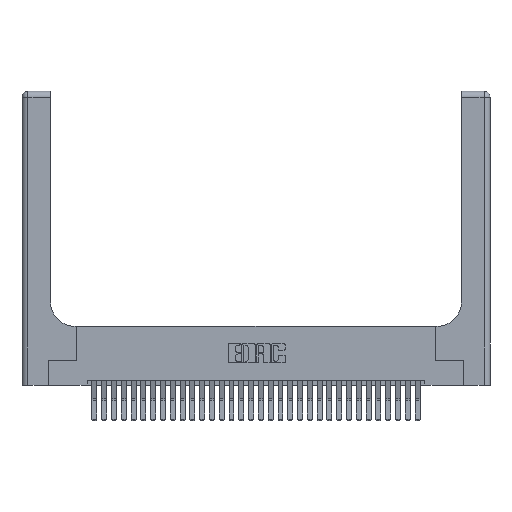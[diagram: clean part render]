
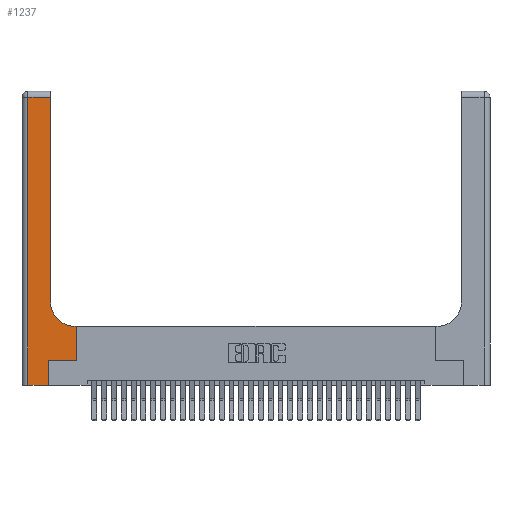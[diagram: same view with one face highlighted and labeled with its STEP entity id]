
A CAD part, top view. The second image highlights one B-rep face of the part: STEP entity #1237.
In plain terms, the highlighted planar face has unit normal (0, 0, 1).
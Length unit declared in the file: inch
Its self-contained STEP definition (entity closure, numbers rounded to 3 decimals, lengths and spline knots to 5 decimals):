
#250 = DIRECTION ( 'NONE',  ( 0., 1., 0. ) ) ;
#1136 = ORIENTED_EDGE ( 'NONE', *, *, #24764, .T. ) ;
#1237 = ADVANCED_FACE ( 'NONE', ( #21443 ), #8126, .F. ) ;
#2355 = CARTESIAN_POINT ( 'NONE',  ( 0.06, 0., 0.37 ) ) ;
#3343 = CARTESIAN_POINT ( 'NONE',  ( 0.06, 3., 0.37 ) ) ;
#3361 = EDGE_CURVE ( 'NONE', #28414, #32316, #3739, .T. ) ;
#3411 = LINE ( 'NONE', #3343, #25801 ) ;
#3739 = LINE ( 'NONE', #21018, #9741 ) ;
#3872 = EDGE_CURVE ( 'NONE', #28305, #20865, #8903, .T. ) ;
#4763 = VERTEX_POINT ( 'NONE', #10488 ) ;
#5432 = VERTEX_POINT ( 'NONE', #10334 ) ;
#5720 = DIRECTION ( 'NONE',  ( -1., 0., 0. ) ) ;
#6015 = EDGE_CURVE ( 'NONE', #20865, #5432, #26299, .T. ) ;
#6050 = LINE ( 'NONE', #10489, #30754 ) ;
#7619 = CARTESIAN_POINT ( 'NONE',  ( 0.269, 0., 0.37 ) ) ;
#7995 = DIRECTION ( 'NONE',  ( -1., 0., 0. ) ) ;
#8056 = DIRECTION ( 'NONE',  ( 0., 0., -1. ) ) ;
#8109 = CIRCLE ( 'NONE', #25505, 0.25 ) ;
#8126 = PLANE ( 'NONE',  #14639 ) ;
#8235 = CARTESIAN_POINT ( 'NONE',  ( 0.5585, 0.25, 0.37 ) ) ;
#8295 = CARTESIAN_POINT ( 'NONE',  ( 0., 3., 0.37 ) ) ;
#8903 = LINE ( 'NONE', #18046, #21658 ) ;
#9468 = ORIENTED_EDGE ( 'NONE', *, *, #23915, .T. ) ;
#9731 = CARTESIAN_POINT ( 'NONE',  ( 0.5585, 0.25, 0.37 ) ) ;
#9741 = VECTOR ( 'NONE', #23598, 39.37008 ) ;
#9792 = ORIENTED_EDGE ( 'NONE', *, *, #22932, .T. ) ;
#10334 = CARTESIAN_POINT ( 'NONE',  ( 0.5585, 0.6, 0.37 ) ) ;
#10488 = CARTESIAN_POINT ( 'NONE',  ( 0.06, 2.94, 0.37 ) ) ;
#10489 = CARTESIAN_POINT ( 'NONE',  ( 0.2915, 3., 0.37 ) ) ;
#12262 = CARTESIAN_POINT ( 'NONE',  ( 0.269, 0.25, 0.37 ) ) ;
#12345 = DIRECTION ( 'NONE',  ( 0., 1., 0. ) ) ;
#12402 = EDGE_LOOP ( 'NONE', ( #27094, #12932, #9468, #13597, #1136, #17725, #28797, #9792, #27145 ) ) ;
#12486 = CARTESIAN_POINT ( 'NONE',  ( 0.2915, 0.85, 0.37 ) ) ;
#12932 = ORIENTED_EDGE ( 'NONE', *, *, #32480, .T. ) ;
#13597 = ORIENTED_EDGE ( 'NONE', *, *, #3361, .T. ) ;
#14222 = CARTESIAN_POINT ( 'NONE',  ( 0.2915, 2.94, 0.37 ) ) ;
#14639 = AXIS2_PLACEMENT_3D ( 'NONE', #8295, #8056, #7995 ) ;
#15144 = DIRECTION ( 'NONE',  ( 0., 0., -1. ) ) ;
#15532 = DIRECTION ( 'NONE',  ( 1., 0., 0. ) ) ;
#16911 = CARTESIAN_POINT ( 'NONE',  ( 0.5415, 0.6, 0.37 ) ) ;
#17421 = VECTOR ( 'NONE', #32781, 39.37008 ) ;
#17451 = CARTESIAN_POINT ( 'NONE',  ( 0.269, 0., 0.37 ) ) ;
#17725 = ORIENTED_EDGE ( 'NONE', *, *, #3872, .T. ) ;
#18046 = CARTESIAN_POINT ( 'NONE',  ( 0.269, 0.25, 0.37 ) ) ;
#18403 = CARTESIAN_POINT ( 'NONE',  ( 0., 2.94, 0.37 ) ) ;
#20865 = VERTEX_POINT ( 'NONE', #8235 ) ;
#21018 = CARTESIAN_POINT ( 'NONE',  ( 0., 0., 0.37 ) ) ;
#21443 = FACE_OUTER_BOUND ( 'NONE', #12402, .T. ) ;
#21658 = VECTOR ( 'NONE', #15532, 39.37008 ) ;
#21734 = VERTEX_POINT ( 'NONE', #14222 ) ;
#22932 = EDGE_CURVE ( 'NONE', #5432, #24723, #30987, .T. ) ;
#23598 = DIRECTION ( 'NONE',  ( 1., 0., 0. ) ) ;
#23786 = DIRECTION ( 'NONE',  ( 0., -1., 0. ) ) ;
#23915 = EDGE_CURVE ( 'NONE', #4763, #28414, #3411, .T. ) ;
#24379 = EDGE_CURVE ( 'NONE', #28365, #21734, #6050, .T. ) ;
#24723 = VERTEX_POINT ( 'NONE', #16911 ) ;
#24764 = EDGE_CURVE ( 'NONE', #32316, #28305, #28005, .T. ) ;
#25493 = VECTOR ( 'NONE', #12345, 39.37008 ) ;
#25505 = AXIS2_PLACEMENT_3D ( 'NONE', #30416, #15144, #32901 ) ;
#25662 = VECTOR ( 'NONE', #5720, 39.37008 ) ;
#25801 = VECTOR ( 'NONE', #23786, 39.37008 ) ;
#26299 = LINE ( 'NONE', #9731, #25493 ) ;
#27094 = ORIENTED_EDGE ( 'NONE', *, *, #24379, .T. ) ;
#27145 = ORIENTED_EDGE ( 'NONE', *, *, #31714, .T. ) ;
#27211 = VECTOR ( 'NONE', #32242, 39.37008 ) ;
#28005 = LINE ( 'NONE', #17451, #27211 ) ;
#28305 = VERTEX_POINT ( 'NONE', #12262 ) ;
#28365 = VERTEX_POINT ( 'NONE', #12486 ) ;
#28414 = VERTEX_POINT ( 'NONE', #2355 ) ;
#28797 = ORIENTED_EDGE ( 'NONE', *, *, #6015, .T. ) ;
#30416 = CARTESIAN_POINT ( 'NONE',  ( 0.5415, 0.85, 0.37 ) ) ;
#30754 = VECTOR ( 'NONE', #250, 39.37008 ) ;
#30987 = LINE ( 'NONE', #32568, #17421 ) ;
#31714 = EDGE_CURVE ( 'NONE', #24723, #28365, #8109, .T. ) ;
#32242 = DIRECTION ( 'NONE',  ( 0., 1., 0. ) ) ;
#32316 = VERTEX_POINT ( 'NONE', #7619 ) ;
#32346 = LINE ( 'NONE', #18403, #25662 ) ;
#32480 = EDGE_CURVE ( 'NONE', #21734, #4763, #32346, .T. ) ;
#32568 = CARTESIAN_POINT ( 'NONE',  ( 0.2915, 0.6, 0.37 ) ) ;
#32781 = DIRECTION ( 'NONE',  ( -1., 0., 0. ) ) ;
#32901 = DIRECTION ( 'NONE',  ( 1., 0., 0. ) ) ;
